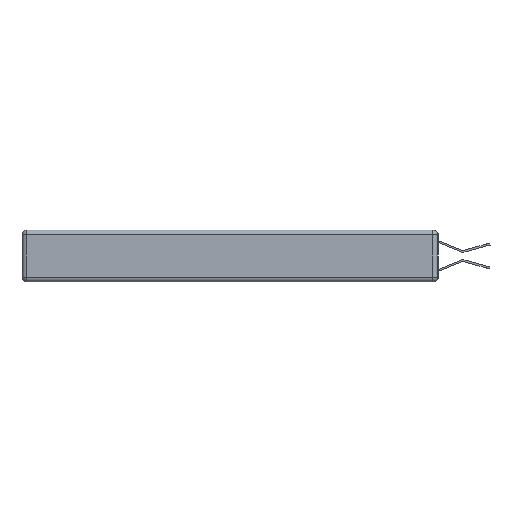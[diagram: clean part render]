
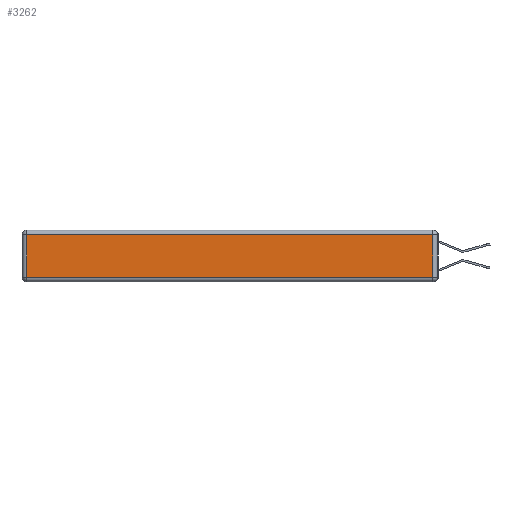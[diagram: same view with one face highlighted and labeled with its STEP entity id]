
A CAD part, left-side view. The second image highlights one B-rep face of the part: STEP entity #3262.
In plain terms, the highlighted planar face has unit normal (-1, 0, 0).
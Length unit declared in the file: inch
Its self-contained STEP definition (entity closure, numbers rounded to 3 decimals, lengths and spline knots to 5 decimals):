
#170 = EDGE_CURVE ( 'NONE', #9277, #3933, #9886, .T. ) ;
#1457 = DIRECTION ( 'NONE',  ( -1., 0., 0. ) ) ;
#2323 = EDGE_CURVE ( 'NONE', #7008, #9277, #9446, .T. ) ;
#3051 = EDGE_CURVE ( 'NONE', #3933, #5161, #12394, .T. ) ;
#3253 = CARTESIAN_POINT ( 'NONE',  ( 0., 2.72, -0.343 ) ) ;
#3262 = ADVANCED_FACE ( 'NONE', ( #11918 ), #3676, .T. ) ;
#3352 = DIRECTION ( 'NONE',  ( 0., 1., 0. ) ) ;
#3676 = PLANE ( 'NONE',  #10076 ) ;
#3879 = CARTESIAN_POINT ( 'NONE',  ( 0., 0.03, -0.343 ) ) ;
#3887 = ORIENTED_EDGE ( 'NONE', *, *, #2323, .T. ) ;
#3933 = VERTEX_POINT ( 'NONE', #6028 ) ;
#4022 = ORIENTED_EDGE ( 'NONE', *, *, #3051, .T. ) ;
#5161 = VERTEX_POINT ( 'NONE', #12134 ) ;
#5631 = ORIENTED_EDGE ( 'NONE', *, *, #170, .T. ) ;
#6028 = CARTESIAN_POINT ( 'NONE',  ( 0., 0.03, -0.313 ) ) ;
#6195 = DIRECTION ( 'NONE',  ( 0., 0., 1. ) ) ;
#6326 = CARTESIAN_POINT ( 'NONE',  ( 0., 2.75, -0.03 ) ) ;
#7008 = VERTEX_POINT ( 'NONE', #8974 ) ;
#7321 = VECTOR ( 'NONE', #13003, 39.37008 ) ;
#7834 = EDGE_LOOP ( 'NONE', ( #5631, #4022, #10431, #3887 ) ) ;
#7897 = VECTOR ( 'NONE', #6195, 39.37008 ) ;
#8849 = CARTESIAN_POINT ( 'NONE',  ( 0., 0., -0.313 ) ) ;
#8974 = CARTESIAN_POINT ( 'NONE',  ( 0., 2.72, -0.03 ) ) ;
#9277 = VERTEX_POINT ( 'NONE', #11330 ) ;
#9446 = LINE ( 'NONE', #3253, #10497 ) ;
#9886 = LINE ( 'NONE', #8849, #7321 ) ;
#10076 = AXIS2_PLACEMENT_3D ( 'NONE', #12857, #1457, #10837 ) ;
#10431 = ORIENTED_EDGE ( 'NONE', *, *, #13311, .T. ) ;
#10497 = VECTOR ( 'NONE', #11554, 39.37008 ) ;
#10580 = LINE ( 'NONE', #6326, #11608 ) ;
#10837 = DIRECTION ( 'NONE',  ( 0., 0., 1. ) ) ;
#11330 = CARTESIAN_POINT ( 'NONE',  ( 0., 2.72, -0.313 ) ) ;
#11554 = DIRECTION ( 'NONE',  ( 0., 0., -1. ) ) ;
#11608 = VECTOR ( 'NONE', #3352, 39.37008 ) ;
#11918 = FACE_OUTER_BOUND ( 'NONE', #7834, .T. ) ;
#12134 = CARTESIAN_POINT ( 'NONE',  ( 0., 0.03, -0.03 ) ) ;
#12394 = LINE ( 'NONE', #3879, #7897 ) ;
#12857 = CARTESIAN_POINT ( 'NONE',  ( 0., 0., -0.343 ) ) ;
#13003 = DIRECTION ( 'NONE',  ( 0., -1., 0. ) ) ;
#13311 = EDGE_CURVE ( 'NONE', #5161, #7008, #10580, .T. ) ;
